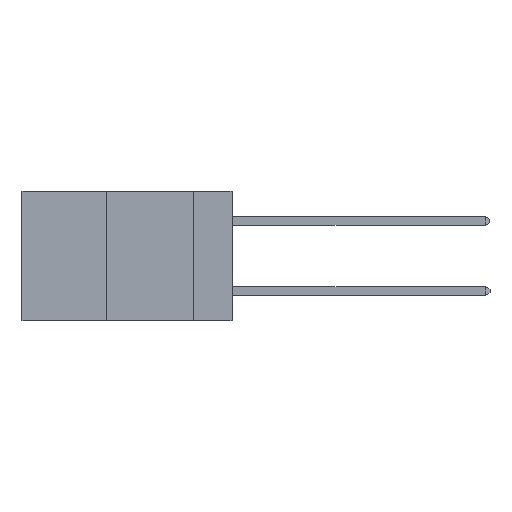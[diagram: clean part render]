
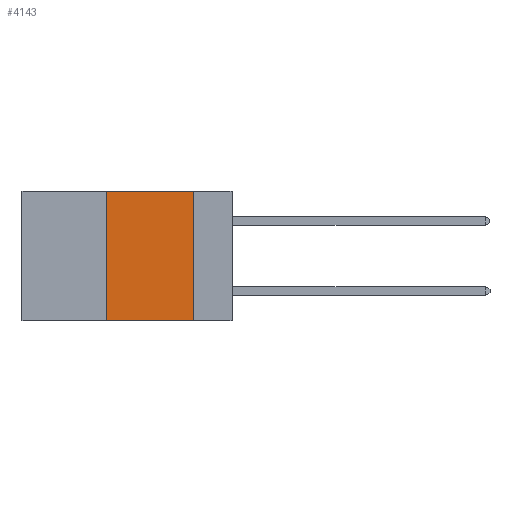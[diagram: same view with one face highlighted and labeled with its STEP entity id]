
A CAD part, left-side view. The second image highlights one B-rep face of the part: STEP entity #4143.
In plain terms, the highlighted planar face has unit normal (-1, 0, 0).
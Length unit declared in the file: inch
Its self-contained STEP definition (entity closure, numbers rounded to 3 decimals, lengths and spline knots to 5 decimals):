
#251 = VECTOR ( 'NONE', #2212, 39.37008 ) ;
#802 = LINE ( 'NONE', #3872, #251 ) ;
#2212 = DIRECTION ( 'NONE',  ( 0., -1., 0. ) ) ;
#2444 = PLANE ( 'NONE',  #15209 ) ;
#3026 = CARTESIAN_POINT ( 'NONE',  ( 0., 0.6, 0. ) ) ;
#3872 = CARTESIAN_POINT ( 'NONE',  ( 0., 0.6, -0.37 ) ) ;
#4143 = ADVANCED_FACE ( 'NONE', ( #16173 ), #2444, .F. ) ;
#4219 = EDGE_LOOP ( 'NONE', ( #17058, #21850, #20318, #6274 ) ) ;
#5160 = VERTEX_POINT ( 'NONE', #18662 ) ;
#5810 = DIRECTION ( 'NONE',  ( 1., 0., 0. ) ) ;
#6274 = ORIENTED_EDGE ( 'NONE', *, *, #6579, .T. ) ;
#6579 = EDGE_CURVE ( 'NONE', #11514, #20363, #802, .T. ) ;
#7648 = DIRECTION ( 'NONE',  ( 0., 0., -1. ) ) ;
#7859 = LINE ( 'NONE', #16082, #11788 ) ;
#8859 = EDGE_CURVE ( 'NONE', #11514, #5160, #21831, .T. ) ;
#9773 = DIRECTION ( 'NONE',  ( 0., -1., 0. ) ) ;
#10742 = VECTOR ( 'NONE', #9773, 39.37008 ) ;
#11514 = VERTEX_POINT ( 'NONE', #14588 ) ;
#11788 = VECTOR ( 'NONE', #7648, 39.37008 ) ;
#12880 = VECTOR ( 'NONE', #15839, 39.37008 ) ;
#14331 = CARTESIAN_POINT ( 'NONE',  ( 0., 0.6, 0. ) ) ;
#14588 = CARTESIAN_POINT ( 'NONE',  ( 0., 0.36, -0.37 ) ) ;
#15033 = EDGE_CURVE ( 'NONE', #5160, #19112, #15299, .T. ) ;
#15209 = AXIS2_PLACEMENT_3D ( 'NONE', #14331, #5810, #17711 ) ;
#15299 = LINE ( 'NONE', #3026, #10742 ) ;
#15839 = DIRECTION ( 'NONE',  ( 0., 0., 1. ) ) ;
#16082 = CARTESIAN_POINT ( 'NONE',  ( 0., 0.11, 0. ) ) ;
#16173 = FACE_OUTER_BOUND ( 'NONE', #4219, .T. ) ;
#16368 = CARTESIAN_POINT ( 'NONE',  ( 0., 0.11, 0. ) ) ;
#17058 = ORIENTED_EDGE ( 'NONE', *, *, #19096, .F. ) ;
#17711 = DIRECTION ( 'NONE',  ( 0., 0., -1. ) ) ;
#18662 = CARTESIAN_POINT ( 'NONE',  ( 0., 0.36, 0. ) ) ;
#19096 = EDGE_CURVE ( 'NONE', #19112, #20363, #7859, .T. ) ;
#19112 = VERTEX_POINT ( 'NONE', #16368 ) ;
#19923 = CARTESIAN_POINT ( 'NONE',  ( 0., 0.11, -0.37 ) ) ;
#20318 = ORIENTED_EDGE ( 'NONE', *, *, #8859, .F. ) ;
#20363 = VERTEX_POINT ( 'NONE', #19923 ) ;
#20811 = CARTESIAN_POINT ( 'NONE',  ( 0., 0.36, 0. ) ) ;
#21831 = LINE ( 'NONE', #20811, #12880 ) ;
#21850 = ORIENTED_EDGE ( 'NONE', *, *, #15033, .F. ) ;
